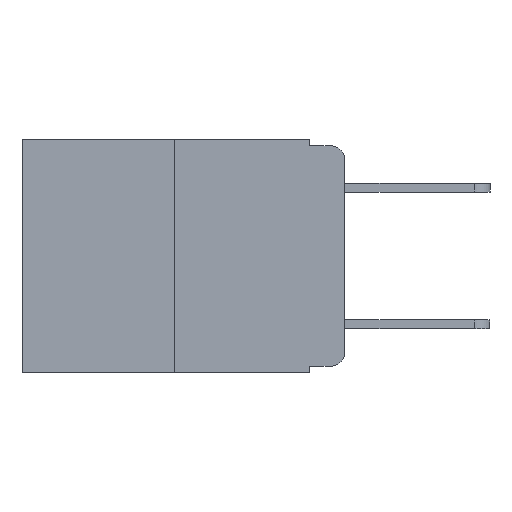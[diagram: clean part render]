
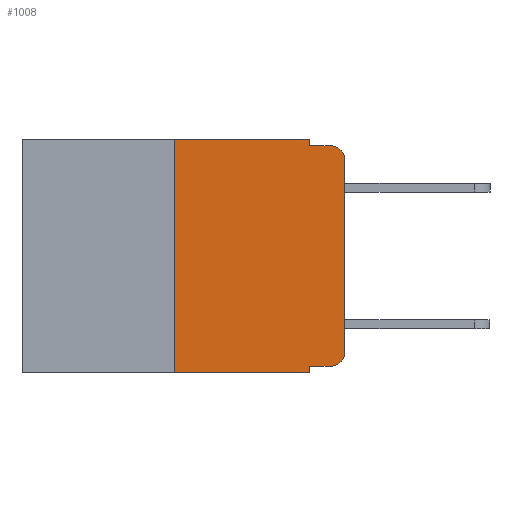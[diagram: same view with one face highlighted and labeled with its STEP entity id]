
A CAD part, left-side view. The second image highlights one B-rep face of the part: STEP entity #1008.
In plain terms, the highlighted planar face has unit normal (-1, 0, 0).
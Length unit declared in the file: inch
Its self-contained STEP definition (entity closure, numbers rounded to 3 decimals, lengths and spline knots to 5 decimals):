
#53 = LINE ( 'NONE', #4076, #13721 ) ;
#209 = DIRECTION ( 'NONE',  ( -1., 0., 0. ) ) ;
#227 = DIRECTION ( 'NONE',  ( 0., -1., 0. ) ) ;
#243 = CARTESIAN_POINT ( 'NONE',  ( 0., 0.25, 0. ) ) ;
#272 = CARTESIAN_POINT ( 'NONE',  ( 0., 0.051, 0. ) ) ;
#341 = VECTOR ( 'NONE', #9930, 39.37008 ) ;
#669 = CARTESIAN_POINT ( 'NONE',  ( 0., 0., 0. ) ) ;
#692 = VERTEX_POINT ( 'NONE', #6850 ) ;
#725 = DIRECTION ( 'NONE',  ( 0., 0., -1. ) ) ;
#943 = ORIENTED_EDGE ( 'NONE', *, *, #13150, .F. ) ;
#971 = CARTESIAN_POINT ( 'NONE',  ( 0., 0.051, -0.01 ) ) ;
#1008 = ADVANCED_FACE ( 'NONE', ( #8720 ), #13847, .F. ) ;
#1198 = EDGE_LOOP ( 'NONE', ( #5510, #4904, #8618, #9070, #8969, #943, #7397, #7589, #7528, #7229 ) ) ;
#1527 = EDGE_CURVE ( 'NONE', #13142, #9485, #10418, .T. ) ;
#1579 = VECTOR ( 'NONE', #6015, 39.37008 ) ;
#1622 = VECTOR ( 'NONE', #227, 39.37008 ) ;
#2330 = AXIS2_PLACEMENT_3D ( 'NONE', #13521, #7716, #725 ) ;
#2370 = EDGE_CURVE ( 'NONE', #9485, #7152, #53, .T. ) ;
#2440 = VECTOR ( 'NONE', #7438, 39.37008 ) ;
#2654 = CIRCLE ( 'NONE', #5960, 0.02 ) ;
#2802 = CARTESIAN_POINT ( 'NONE',  ( 0., 0.051, 0. ) ) ;
#2969 = LINE ( 'NONE', #3000, #13669 ) ;
#3000 = CARTESIAN_POINT ( 'NONE',  ( 0., 0.051, -0.333 ) ) ;
#3901 = EDGE_CURVE ( 'NONE', #12803, #7152, #2654, .T. ) ;
#4043 = CARTESIAN_POINT ( 'NONE',  ( 0., 0.051, 0. ) ) ;
#4076 = CARTESIAN_POINT ( 'NONE',  ( 0., 0.051, -0.01 ) ) ;
#4219 = DIRECTION ( 'NONE',  ( 0., 0., -1. ) ) ;
#4244 = DIRECTION ( 'NONE',  ( 1., 0., 0. ) ) ;
#4259 = VECTOR ( 'NONE', #13526, 39.37008 ) ;
#4469 = VERTEX_POINT ( 'NONE', #8550 ) ;
#4714 = CARTESIAN_POINT ( 'NONE',  ( 0., 0.02, -0.01 ) ) ;
#4904 = ORIENTED_EDGE ( 'NONE', *, *, #3901, .T. ) ;
#4926 = CARTESIAN_POINT ( 'NONE',  ( 0., 0.02, -0.03 ) ) ;
#5268 = VECTOR ( 'NONE', #6241, 39.37008 ) ;
#5510 = ORIENTED_EDGE ( 'NONE', *, *, #6913, .T. ) ;
#5559 = AXIS2_PLACEMENT_3D ( 'NONE', #8490, #4244, #12846 ) ;
#5625 = CARTESIAN_POINT ( 'NONE',  ( 0., 0.25, -0.343 ) ) ;
#5652 = DIRECTION ( 'NONE',  ( 0., -1., 0. ) ) ;
#5698 = VERTEX_POINT ( 'NONE', #13780 ) ;
#5960 = AXIS2_PLACEMENT_3D ( 'NONE', #4926, #209, #4219 ) ;
#6015 = DIRECTION ( 'NONE',  ( 0., 0., -1. ) ) ;
#6241 = DIRECTION ( 'NONE',  ( 0., 0., 1. ) ) ;
#6360 = VERTEX_POINT ( 'NONE', #12673 ) ;
#6429 = DIRECTION ( 'NONE',  ( 0., -1., 0. ) ) ;
#6664 = LINE ( 'NONE', #8878, #341 ) ;
#6838 = VERTEX_POINT ( 'NONE', #12493 ) ;
#6850 = CARTESIAN_POINT ( 'NONE',  ( 0., 0.051, -0.333 ) ) ;
#6913 = EDGE_CURVE ( 'NONE', #4469, #12803, #7602, .T. ) ;
#7152 = VERTEX_POINT ( 'NONE', #4714 ) ;
#7229 = ORIENTED_EDGE ( 'NONE', *, *, #11279, .T. ) ;
#7397 = ORIENTED_EDGE ( 'NONE', *, *, #13898, .T. ) ;
#7438 = DIRECTION ( 'NONE',  ( 0., 0., -1. ) ) ;
#7528 = ORIENTED_EDGE ( 'NONE', *, *, #11937, .T. ) ;
#7589 = ORIENTED_EDGE ( 'NONE', *, *, #12553, .F. ) ;
#7602 = LINE ( 'NONE', #669, #4259 ) ;
#7716 = DIRECTION ( 'NONE',  ( -1., 0., 0. ) ) ;
#8076 = LINE ( 'NONE', #8428, #1622 ) ;
#8251 = LINE ( 'NONE', #243, #5268 ) ;
#8428 = CARTESIAN_POINT ( 'NONE',  ( 0., 0.473, 0. ) ) ;
#8442 = LINE ( 'NONE', #4043, #2440 ) ;
#8490 = CARTESIAN_POINT ( 'NONE',  ( 0., 0.473, 0. ) ) ;
#8550 = CARTESIAN_POINT ( 'NONE',  ( 0., 0., -0.313 ) ) ;
#8618 = ORIENTED_EDGE ( 'NONE', *, *, #2370, .F. ) ;
#8720 = FACE_OUTER_BOUND ( 'NONE', #1198, .T. ) ;
#8789 = EDGE_CURVE ( 'NONE', #6360, #13142, #8076, .T. ) ;
#8878 = CARTESIAN_POINT ( 'NONE',  ( 0., 0.473, -0.343 ) ) ;
#8969 = ORIENTED_EDGE ( 'NONE', *, *, #8789, .F. ) ;
#9070 = ORIENTED_EDGE ( 'NONE', *, *, #1527, .F. ) ;
#9408 = CIRCLE ( 'NONE', #2330, 0.02 ) ;
#9485 = VERTEX_POINT ( 'NONE', #971 ) ;
#9930 = DIRECTION ( 'NONE',  ( 0., -1., 0. ) ) ;
#10418 = LINE ( 'NONE', #272, #1579 ) ;
#11279 = EDGE_CURVE ( 'NONE', #6838, #4469, #9408, .T. ) ;
#11828 = CARTESIAN_POINT ( 'NONE',  ( 0., 0., -0.03 ) ) ;
#11937 = EDGE_CURVE ( 'NONE', #692, #6838, #2969, .T. ) ;
#12493 = CARTESIAN_POINT ( 'NONE',  ( 0., 0.02, -0.333 ) ) ;
#12553 = EDGE_CURVE ( 'NONE', #692, #5698, #8442, .T. ) ;
#12673 = CARTESIAN_POINT ( 'NONE',  ( 0., 0.25, 0. ) ) ;
#12802 = VERTEX_POINT ( 'NONE', #5625 ) ;
#12803 = VERTEX_POINT ( 'NONE', #11828 ) ;
#12846 = DIRECTION ( 'NONE',  ( 0., 0., -1. ) ) ;
#13142 = VERTEX_POINT ( 'NONE', #2802 ) ;
#13150 = EDGE_CURVE ( 'NONE', #12802, #6360, #8251, .T. ) ;
#13521 = CARTESIAN_POINT ( 'NONE',  ( 0., 0.02, -0.313 ) ) ;
#13526 = DIRECTION ( 'NONE',  ( 0., 0., 1. ) ) ;
#13669 = VECTOR ( 'NONE', #6429, 39.37008 ) ;
#13721 = VECTOR ( 'NONE', #5652, 39.37008 ) ;
#13780 = CARTESIAN_POINT ( 'NONE',  ( 0., 0.051, -0.343 ) ) ;
#13847 = PLANE ( 'NONE',  #5559 ) ;
#13898 = EDGE_CURVE ( 'NONE', #12802, #5698, #6664, .T. ) ;
